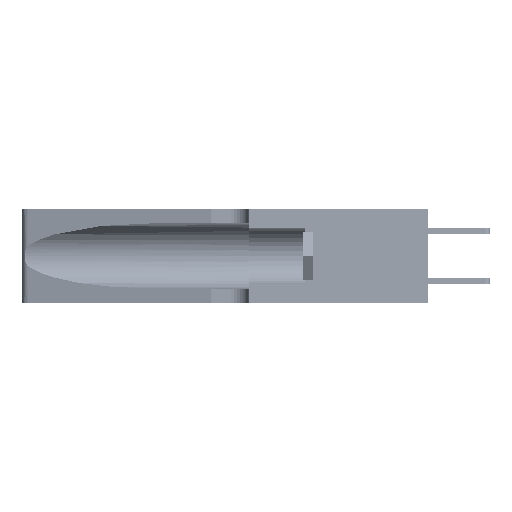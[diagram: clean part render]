
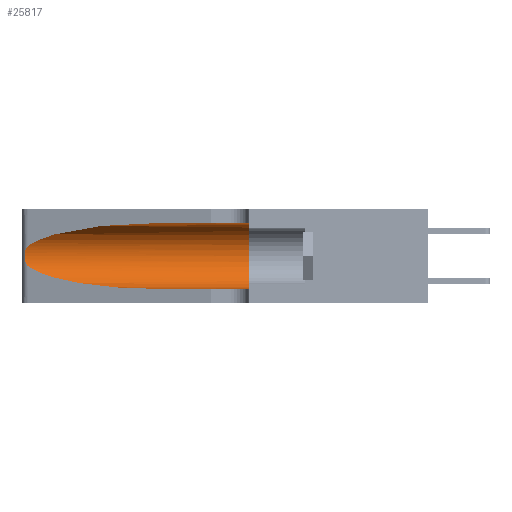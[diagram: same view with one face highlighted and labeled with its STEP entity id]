
A CAD part, left-side view. The second image highlights one B-rep face of the part: STEP entity #25817.
In plain terms, the highlighted cylindrical face has radius 3.308 mm (diameter 6.617 mm), a partial arc.
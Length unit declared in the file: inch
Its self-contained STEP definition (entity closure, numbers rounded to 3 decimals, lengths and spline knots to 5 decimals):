
#116 = VECTOR ( 'NONE', #28141, 39.37008 ) ;
#382 = CARTESIAN_POINT ( 'NONE',  ( 0.1305, 1.61858, 0.185 ) ) ;
#546 = VERTEX_POINT ( 'NONE', #24526 ) ;
#2494 = CARTESIAN_POINT ( 'NONE',  ( 0.25487, 1.22718, 0.22369 ) ) ;
#2659 = CARTESIAN_POINT ( 'NONE',  ( 0.1305, 1.61858, 0.05475 ) ) ;
#3378 = DIRECTION ( 'NONE',  ( 0., -1., 0. ) ) ;
#4258 = DIRECTION ( 'NONE',  ( 0., 1., 0. ) ) ;
#4334 = AXIS2_PLACEMENT_3D ( 'NONE', #45820, #4258, #41773 ) ;
#6310 = CARTESIAN_POINT ( 'NONE',  ( 0.26018, 1.23835, 0.19895 ) ) ;
#6323 = VERTEX_POINT ( 'NONE', #25922 ) ;
#9997 = CARTESIAN_POINT ( 'NONE',  ( 0.25854, 1.2359, 0.20912 ) ) ;
#10174 = CARTESIAN_POINT ( 'NONE',  ( 0.25787, 1.23484, 0.2124 ) ) ;
#11486 = CARTESIAN_POINT ( 'NONE',  ( 0.1305, 1.61858, 0.31525 ) ) ;
#11717 = EDGE_CURVE ( 'NONE', #34024, #20072, #29793, .T. ) ;
#13014 = EDGE_CURVE ( 'NONE', #33097, #6323, #23928, .T. ) ;
#14443 = ORIENTED_EDGE ( 'NONE', *, *, #13014, .F. ) ;
#14971 = VERTEX_POINT ( 'NONE', #49145 ) ;
#15709 = CARTESIAN_POINT ( 'NONE',  ( 0.25487, 1.22718, 0.14631 ) ) ;
#15787 = CYLINDRICAL_SURFACE ( 'NONE', #53148, 0.13025 ) ;
#17176 = CARTESIAN_POINT ( 'NONE',  ( 0.25487, 1.22718, 0.22369 ) ) ;
#17901 = DIRECTION ( 'NONE',  ( 0., 0., -1. ) ) ;
#19226 =( BOUNDED_CURVE ( )  B_SPLINE_CURVE ( 3, ( #21964, #47115, #42689, #17176 ),
 .UNSPECIFIED., .F., .F. ) 
 B_SPLINE_CURVE_WITH_KNOTS ( ( 4, 4 ),
 ( 1.5708, 2.84003 ),
 .UNSPECIFIED. ) 
 CURVE ( )  GEOMETRIC_REPRESENTATION_ITEM ( )  RATIONAL_B_SPLINE_CURVE ( ( 1., 0.87, 0.87, 1. ) ) 
 REPRESENTATION_ITEM ( '' )  );
#20072 = VERTEX_POINT ( 'NONE', #15709 ) ;
#20605 = LINE ( 'NONE', #2659, #116 ) ;
#21964 = CARTESIAN_POINT ( 'NONE',  ( 0.1305, 0.72297, 0.31525 ) ) ;
#22538 = CARTESIAN_POINT ( 'NONE',  ( 0.26075, 1.23896, 0.178 ) ) ;
#23081 = CARTESIAN_POINT ( 'NONE',  ( 0.25555, 1.22994, 0.2215 ) ) ;
#23928 = LINE ( 'NONE', #11486, #37849 ) ;
#24241 = EDGE_CURVE ( 'NONE', #14971, #546, #20605, .T. ) ;
#24526 = CARTESIAN_POINT ( 'NONE',  ( 0.1305, 0.35, 0.05475 ) ) ;
#25817 = ADVANCED_FACE ( 'NONE', ( #44843 ), #15787, .F. ) ;
#25922 = CARTESIAN_POINT ( 'NONE',  ( 0.1305, 0.35, 0.31525 ) ) ;
#26401 = EDGE_CURVE ( 'NONE', #20072, #14971, #45319, .T. ) ;
#26809 = CARTESIAN_POINT ( 'NONE',  ( 0.25789, 1.23486, 0.15765 ) ) ;
#27178 = CARTESIAN_POINT ( 'NONE',  ( 0.25639, 1.23186, 0.15144 ) ) ;
#27244 = ORIENTED_EDGE ( 'NONE', *, *, #24241, .T. ) ;
#28141 = DIRECTION ( 'NONE',  ( 0., -1., 0. ) ) ;
#29146 = CARTESIAN_POINT ( 'NONE',  ( 0.25487, 1.22718, 0.14631 ) ) ;
#29793 = B_SPLINE_CURVE_WITH_KNOTS ( 'NONE', 3,
 ( #31267, #23081, #47858, #10174, #9997, #6310, #43979, #22538, #35660, #52115, #26809, #27178, #31091, #48219 ),
 .UNSPECIFIED., .F., .F.,
 ( 4, 2, 2, 2, 2, 2, 4 ),
 ( 0., 0.00027, 0.00053, 0.00107, 0.0016, 0.00187, 0.00214 ),
 .UNSPECIFIED. ) ;
#29881 = CARTESIAN_POINT ( 'NONE',  ( 0.2373, 1.15595, 0.08982 ) ) ;
#30584 = EDGE_LOOP ( 'NONE', ( #38507, #45895, #32137, #27244, #32663, #14443 ) ) ;
#31091 = CARTESIAN_POINT ( 'NONE',  ( 0.25555, 1.22993, 0.14849 ) ) ;
#31267 = CARTESIAN_POINT ( 'NONE',  ( 0.25487, 1.22718, 0.22369 ) ) ;
#32137 = ORIENTED_EDGE ( 'NONE', *, *, #26401, .T. ) ;
#32663 = ORIENTED_EDGE ( 'NONE', *, *, #36951, .F. ) ;
#33097 = VERTEX_POINT ( 'NONE', #33640 ) ;
#33640 = CARTESIAN_POINT ( 'NONE',  ( 0.1305, 0.72297, 0.31525 ) ) ;
#34024 = VERTEX_POINT ( 'NONE', #2494 ) ;
#35660 = CARTESIAN_POINT ( 'NONE',  ( 0.26017, 1.23833, 0.17102 ) ) ;
#36951 = EDGE_CURVE ( 'NONE', #6323, #546, #41549, .T. ) ;
#37849 = VECTOR ( 'NONE', #3378, 39.37008 ) ;
#38507 = ORIENTED_EDGE ( 'NONE', *, *, #44143, .T. ) ;
#41549 = CIRCLE ( 'NONE', #4334, 0.13025 ) ;
#41773 = DIRECTION ( 'NONE',  ( 0., 0., 1. ) ) ;
#42500 = DIRECTION ( 'NONE',  ( 0., -1., 0. ) ) ;
#42608 = CARTESIAN_POINT ( 'NONE',  ( 0.18966, 0.96281, 0.05475 ) ) ;
#42689 = CARTESIAN_POINT ( 'NONE',  ( 0.2373, 1.15595, 0.28018 ) ) ;
#43979 = CARTESIAN_POINT ( 'NONE',  ( 0.26075, 1.23896, 0.19203 ) ) ;
#44143 = EDGE_CURVE ( 'NONE', #33097, #34024, #19226, .T. ) ;
#44843 = FACE_OUTER_BOUND ( 'NONE', #30584, .T. ) ;
#45319 =( BOUNDED_CURVE ( )  B_SPLINE_CURVE ( 3, ( #29146, #29881, #42608, #45925 ),
 .UNSPECIFIED., .F., .F. ) 
 B_SPLINE_CURVE_WITH_KNOTS ( ( 4, 4 ),
 ( 3.44316, 4.71239 ),
 .UNSPECIFIED. ) 
 CURVE ( )  GEOMETRIC_REPRESENTATION_ITEM ( )  RATIONAL_B_SPLINE_CURVE ( ( 1., 0.87, 0.87, 1. ) ) 
 REPRESENTATION_ITEM ( '' )  );
#45820 = CARTESIAN_POINT ( 'NONE',  ( 0.1305, 0.35, 0.185 ) ) ;
#45895 = ORIENTED_EDGE ( 'NONE', *, *, #11717, .T. ) ;
#45925 = CARTESIAN_POINT ( 'NONE',  ( 0.1305, 0.72297, 0.05475 ) ) ;
#47115 = CARTESIAN_POINT ( 'NONE',  ( 0.18966, 0.96281, 0.31525 ) ) ;
#47858 = CARTESIAN_POINT ( 'NONE',  ( 0.25639, 1.23184, 0.21858 ) ) ;
#48219 = CARTESIAN_POINT ( 'NONE',  ( 0.25487, 1.22718, 0.14631 ) ) ;
#49145 = CARTESIAN_POINT ( 'NONE',  ( 0.1305, 0.72297, 0.05475 ) ) ;
#52115 = CARTESIAN_POINT ( 'NONE',  ( 0.25856, 1.23593, 0.16098 ) ) ;
#53148 = AXIS2_PLACEMENT_3D ( 'NONE', #382, #42500, #17901 ) ;
